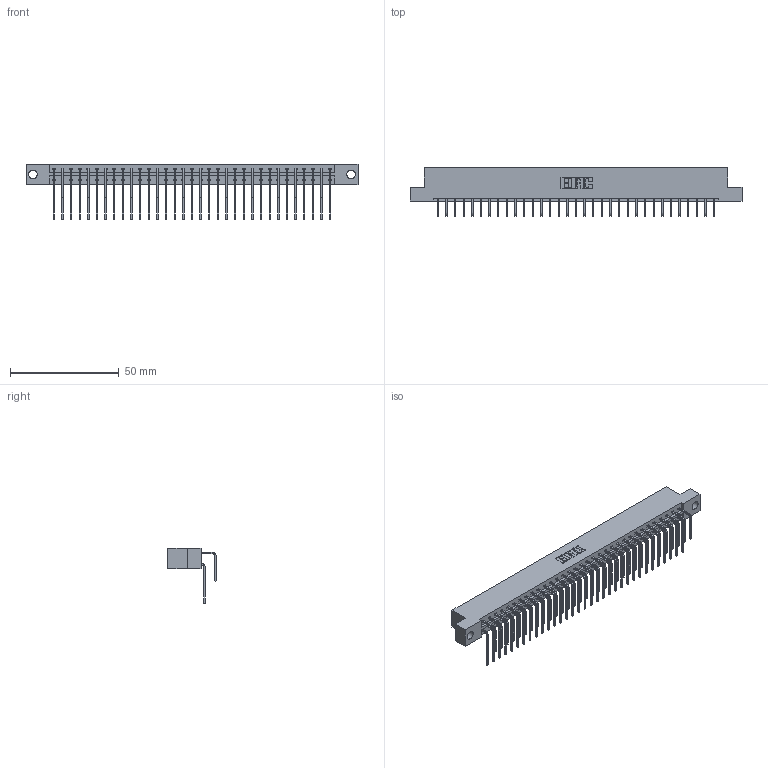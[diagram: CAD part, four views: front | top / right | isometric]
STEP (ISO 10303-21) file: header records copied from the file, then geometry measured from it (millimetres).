
FILE_DESCRIPTION (( 'STEP AP203' ), '1' );
FILE_NAME ('833-066-558-204.STEP', '2020-06-05T09:34:46', ( '' ), ( '' ), 'SwSTEP 2.0', 'SolidWorks 2020', '' );
FILE_SCHEMA (( 'CONFIG_CONTROL_DESIGN' ));
Length unit declared in the file: inch
Products named in the file (4): 345-292-001_558 Tail - 2; 345-292-001_558 559 Tail - 1; 833-066-558-204; 833 Part_Flush - .156 Dia - TH
Assembly tree (67 placements, depth 2):
  833-066-558-204
    833 Part_Flush - .156 Dia - TH
    345-292-001_558 559 Tail - 1  x33
    345-292-001_558 Tail - 2  x33
Bounding box: 152.3 x 22.17 x 25.53 mm (x, y, z)
Volume: 15757.5 mm3; surface area: 20228.5 mm2
Topology: 67 solids, 67 shells, 3678 faces, 10937 edges, 7202 vertices
Faces by surface type: plane 2578, cylinder 1100
Entity records: 24181 total; most frequent: CARTESIAN_POINT 4069, ORIENTED_EDGE 3954, DIRECTION 3473, EDGE_CURVE 1977, LINE 1809, VECTOR 1809, VERTEX_POINT 1314, AXIS2_PLACEMENT_3D 832
